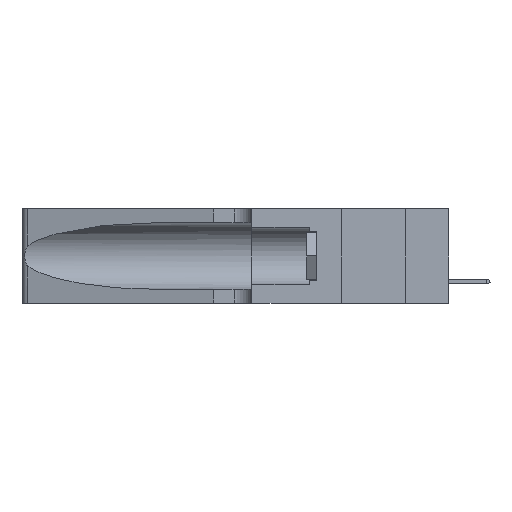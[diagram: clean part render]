
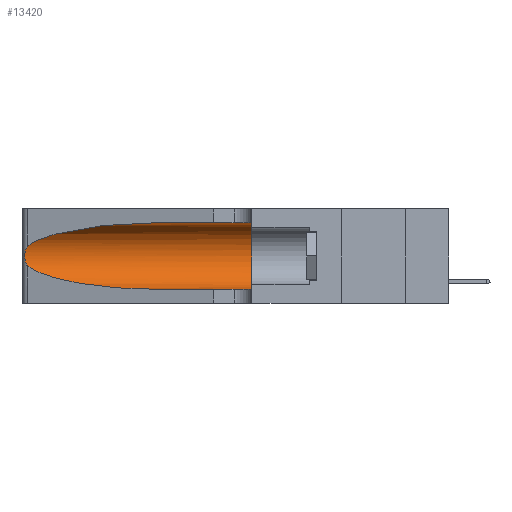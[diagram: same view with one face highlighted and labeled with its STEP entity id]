
A CAD part, left-side view. The second image highlights one B-rep face of the part: STEP entity #13420.
In plain terms, the highlighted cylindrical face has radius 3.308 mm (diameter 6.617 mm), a partial arc.
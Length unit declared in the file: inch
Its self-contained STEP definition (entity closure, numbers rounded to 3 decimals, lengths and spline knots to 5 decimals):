
#957 = ORIENTED_EDGE ( 'NONE', *, *, #44220, .T. ) ;
#1088 = ORIENTED_EDGE ( 'NONE', *, *, #27816, .F. ) ;
#1905 = CARTESIAN_POINT ( 'NONE',  ( 0.26018, 1.23835, 0.19895 ) ) ;
#2993 = CARTESIAN_POINT ( 'NONE',  ( 0.1305, 0.35, 0.185 ) ) ;
#3350 = EDGE_LOOP ( 'NONE', ( #957, #36880, #18750, #42489, #1088, #25107 ) ) ;
#3436 = CARTESIAN_POINT ( 'NONE',  ( 0.25555, 1.22993, 0.14849 ) ) ;
#3457 = VERTEX_POINT ( 'NONE', #9287 ) ;
#4626 = CIRCLE ( 'NONE', #11037, 0.13025 ) ;
#5069 = CARTESIAN_POINT ( 'NONE',  ( 0.26017, 1.23833, 0.17102 ) ) ;
#5306 = CARTESIAN_POINT ( 'NONE',  ( 0.18966, 0.96281, 0.31525 ) ) ;
#5382 = CARTESIAN_POINT ( 'NONE',  ( 0.25487, 1.22718, 0.14631 ) ) ;
#5667 = CARTESIAN_POINT ( 'NONE',  ( 0.1305, 0.72297, 0.05475 ) ) ;
#5797 = AXIS2_PLACEMENT_3D ( 'NONE', #28235, #35610, #8003 ) ;
#6359 = CARTESIAN_POINT ( 'NONE',  ( 0.26075, 1.23896, 0.19203 ) ) ;
#6560 = CARTESIAN_POINT ( 'NONE',  ( 0.1305, 0.72297, 0.05475 ) ) ;
#7419 = DIRECTION ( 'NONE',  ( 0., -1., 0. ) ) ;
#7944 = CARTESIAN_POINT ( 'NONE',  ( 0.25787, 1.23484, 0.2124 ) ) ;
#8003 = DIRECTION ( 'NONE',  ( 0., 0., -1. ) ) ;
#8394 = VERTEX_POINT ( 'NONE', #5667 ) ;
#8809 = CARTESIAN_POINT ( 'NONE',  ( 0.1305, 0.72297, 0.31525 ) ) ;
#9287 = CARTESIAN_POINT ( 'NONE',  ( 0.1305, 0.35, 0.31525 ) ) ;
#11037 = AXIS2_PLACEMENT_3D ( 'NONE', #2993, #39087, #38363 ) ;
#11155 = CARTESIAN_POINT ( 'NONE',  ( 0.2373, 1.15595, 0.08982 ) ) ;
#11905 = CARTESIAN_POINT ( 'NONE',  ( 0.25555, 1.22994, 0.2215 ) ) ;
#13136 = VERTEX_POINT ( 'NONE', #5382 ) ;
#13420 = ADVANCED_FACE ( 'NONE', ( #33665 ), #32572, .F. ) ;
#14783 = EDGE_CURVE ( 'NONE', #8394, #17509, #33238, .T. ) ;
#17225 = CARTESIAN_POINT ( 'NONE',  ( 0.1305, 0.35, 0.05475 ) ) ;
#17509 = VERTEX_POINT ( 'NONE', #17225 ) ;
#17761 = CARTESIAN_POINT ( 'NONE',  ( 0.25487, 1.22718, 0.14631 ) ) ;
#18712 = CARTESIAN_POINT ( 'NONE',  ( 0.25487, 1.22718, 0.22369 ) ) ;
#18750 = ORIENTED_EDGE ( 'NONE', *, *, #37119, .T. ) ;
#20577 = CARTESIAN_POINT ( 'NONE',  ( 0.25639, 1.23186, 0.15144 ) ) ;
#22344 = CARTESIAN_POINT ( 'NONE',  ( 0.25789, 1.23486, 0.15765 ) ) ;
#22866 = EDGE_CURVE ( 'NONE', #41586, #3457, #29061, .T. ) ;
#23419 = B_SPLINE_CURVE_WITH_KNOTS ( 'NONE', 3,
 ( #42463, #11905, #31831, #7944, #23459, #1905, #6359, #39769, #5069, #36010, #22344, #20577, #3436, #41429 ),
 .UNSPECIFIED., .F., .F.,
 ( 4, 2, 2, 2, 2, 2, 4 ),
 ( 0., 0.00027, 0.00053, 0.00107, 0.0016, 0.00187, 0.00214 ),
 .UNSPECIFIED. ) ;
#23459 = CARTESIAN_POINT ( 'NONE',  ( 0.25854, 1.2359, 0.20912 ) ) ;
#23569 = VECTOR ( 'NONE', #39155, 39.37008 ) ;
#25107 = ORIENTED_EDGE ( 'NONE', *, *, #22866, .F. ) ;
#27816 = EDGE_CURVE ( 'NONE', #3457, #17509, #4626, .T. ) ;
#28020 =( BOUNDED_CURVE ( )  B_SPLINE_CURVE ( 3, ( #17761, #11155, #44056, #6560 ),
 .UNSPECIFIED., .F., .F. ) 
 B_SPLINE_CURVE_WITH_KNOTS ( ( 4, 4 ),
 ( 3.44316, 4.71239 ),
 .UNSPECIFIED. ) 
 CURVE ( )  GEOMETRIC_REPRESENTATION_ITEM ( )  RATIONAL_B_SPLINE_CURVE ( ( 1., 0.87, 0.87, 1. ) ) 
 REPRESENTATION_ITEM ( '' )  );
#28235 = CARTESIAN_POINT ( 'NONE',  ( 0.1305, 1.61858, 0.185 ) ) ;
#29061 = LINE ( 'NONE', #38594, #37183 ) ;
#29333 = CARTESIAN_POINT ( 'NONE',  ( 0.2373, 1.15595, 0.28018 ) ) ;
#29999 = EDGE_CURVE ( 'NONE', #43536, #13136, #23419, .T. ) ;
#31831 = CARTESIAN_POINT ( 'NONE',  ( 0.25639, 1.23184, 0.21858 ) ) ;
#32572 = CYLINDRICAL_SURFACE ( 'NONE', #5797, 0.13025 ) ;
#33238 = LINE ( 'NONE', #35724, #23569 ) ;
#33254 = CARTESIAN_POINT ( 'NONE',  ( 0.25487, 1.22718, 0.22369 ) ) ;
#33665 = FACE_OUTER_BOUND ( 'NONE', #3350, .T. ) ;
#35610 = DIRECTION ( 'NONE',  ( 0., -1., 0. ) ) ;
#35724 = CARTESIAN_POINT ( 'NONE',  ( 0.1305, 1.61858, 0.05475 ) ) ;
#36010 = CARTESIAN_POINT ( 'NONE',  ( 0.25856, 1.23593, 0.16098 ) ) ;
#36880 = ORIENTED_EDGE ( 'NONE', *, *, #29999, .T. ) ;
#37119 = EDGE_CURVE ( 'NONE', #13136, #8394, #28020, .T. ) ;
#37183 = VECTOR ( 'NONE', #7419, 39.37008 ) ;
#38363 = DIRECTION ( 'NONE',  ( 0., 0., 1. ) ) ;
#38594 = CARTESIAN_POINT ( 'NONE',  ( 0.1305, 1.61858, 0.31525 ) ) ;
#39037 = CARTESIAN_POINT ( 'NONE',  ( 0.1305, 0.72297, 0.31525 ) ) ;
#39087 = DIRECTION ( 'NONE',  ( 0., 1., 0. ) ) ;
#39155 = DIRECTION ( 'NONE',  ( 0., -1., 0. ) ) ;
#39769 = CARTESIAN_POINT ( 'NONE',  ( 0.26075, 1.23896, 0.178 ) ) ;
#41429 = CARTESIAN_POINT ( 'NONE',  ( 0.25487, 1.22718, 0.14631 ) ) ;
#41586 = VERTEX_POINT ( 'NONE', #39037 ) ;
#42463 = CARTESIAN_POINT ( 'NONE',  ( 0.25487, 1.22718, 0.22369 ) ) ;
#42489 = ORIENTED_EDGE ( 'NONE', *, *, #14783, .T. ) ;
#42626 =( BOUNDED_CURVE ( )  B_SPLINE_CURVE ( 3, ( #8809, #5306, #29333, #33254 ),
 .UNSPECIFIED., .F., .F. ) 
 B_SPLINE_CURVE_WITH_KNOTS ( ( 4, 4 ),
 ( 1.5708, 2.84003 ),
 .UNSPECIFIED. ) 
 CURVE ( )  GEOMETRIC_REPRESENTATION_ITEM ( )  RATIONAL_B_SPLINE_CURVE ( ( 1., 0.87, 0.87, 1. ) ) 
 REPRESENTATION_ITEM ( '' )  );
#43536 = VERTEX_POINT ( 'NONE', #18712 ) ;
#44056 = CARTESIAN_POINT ( 'NONE',  ( 0.18966, 0.96281, 0.05475 ) ) ;
#44220 = EDGE_CURVE ( 'NONE', #41586, #43536, #42626, .T. ) ;
